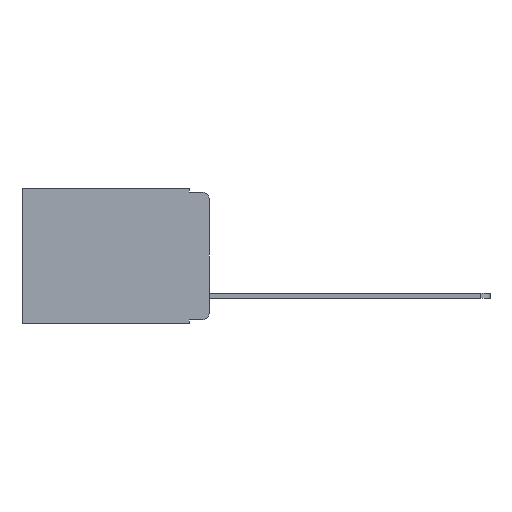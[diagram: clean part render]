
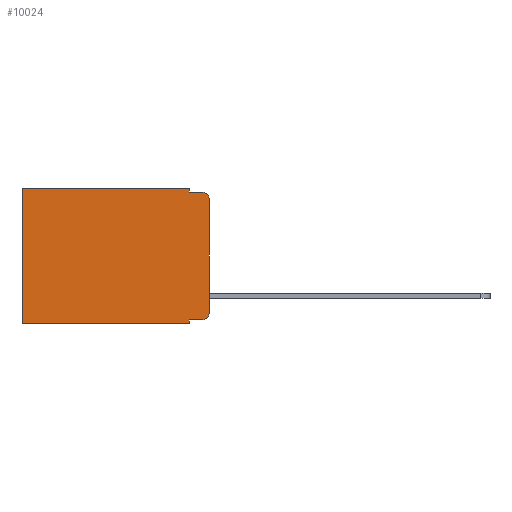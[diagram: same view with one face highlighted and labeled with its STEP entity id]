
A CAD part, left-side view. The second image highlights one B-rep face of the part: STEP entity #10024.
In plain terms, the highlighted planar face has unit normal (-1, 0, 0).
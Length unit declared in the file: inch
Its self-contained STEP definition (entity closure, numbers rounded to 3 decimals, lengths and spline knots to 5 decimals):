
#4 = CARTESIAN_POINT ( 'NONE',  ( 0.298, 0.051, 0. ) ) ;
#123 = VECTOR ( 'NONE', #8739, 39.37008 ) ;
#331 = VECTOR ( 'NONE', #14631, 39.37008 ) ;
#463 = EDGE_CURVE ( 'NONE', #11178, #8515, #7495, .T. ) ;
#680 = VECTOR ( 'NONE', #14620, 39.37008 ) ;
#747 = CARTESIAN_POINT ( 'NONE',  ( 0.298, 0., -0.343 ) ) ;
#1091 = PLANE ( 'NONE',  #6330 ) ;
#1184 = VERTEX_POINT ( 'NONE', #7296 ) ;
#1801 = CARTESIAN_POINT ( 'NONE',  ( 0.298, 0.051, -0.01 ) ) ;
#1900 = DIRECTION ( 'NONE',  ( 0., -1., 0. ) ) ;
#2019 = EDGE_CURVE ( 'NONE', #13394, #2105, #8892, .T. ) ;
#2105 = VERTEX_POINT ( 'NONE', #9127 ) ;
#2339 = VERTEX_POINT ( 'NONE', #5943 ) ;
#2523 = CARTESIAN_POINT ( 'NONE',  ( 0.298, 0.02, -0.333 ) ) ;
#2539 = CARTESIAN_POINT ( 'NONE',  ( 0.298, 0.02, -0.313 ) ) ;
#2757 = CARTESIAN_POINT ( 'NONE',  ( 0.298, 0.473, -0.343 ) ) ;
#3303 = LINE ( 'NONE', #16469, #123 ) ;
#3375 = CARTESIAN_POINT ( 'NONE',  ( 0.298, 0.02, -0.01 ) ) ;
#3895 = DIRECTION ( 'NONE',  ( -1., 0., 0. ) ) ;
#3957 = AXIS2_PLACEMENT_3D ( 'NONE', #2539, #11661, #5196 ) ;
#4052 = CARTESIAN_POINT ( 'NONE',  ( 0.298, 0.02, -0.03 ) ) ;
#4305 = ORIENTED_EDGE ( 'NONE', *, *, #14513, .F. ) ;
#4459 = ORIENTED_EDGE ( 'NONE', *, *, #8218, .F. ) ;
#4557 = EDGE_CURVE ( 'NONE', #2339, #11704, #7590, .T. ) ;
#4608 = EDGE_CURVE ( 'NONE', #1184, #13394, #10288, .T. ) ;
#4707 = ORIENTED_EDGE ( 'NONE', *, *, #5988, .F. ) ;
#4708 = ORIENTED_EDGE ( 'NONE', *, *, #463, .T. ) ;
#4729 = LINE ( 'NONE', #15490, #11447 ) ;
#5196 = DIRECTION ( 'NONE',  ( 0., 0., -1. ) ) ;
#5606 = CARTESIAN_POINT ( 'NONE',  ( 0.298, 0., 0. ) ) ;
#5815 = CARTESIAN_POINT ( 'NONE',  ( 0.298, 0.051, -0.333 ) ) ;
#5943 = CARTESIAN_POINT ( 'NONE',  ( 0.298, 0.051, -0.343 ) ) ;
#5988 = EDGE_CURVE ( 'NONE', #11178, #2105, #3303, .T. ) ;
#6045 = DIRECTION ( 'NONE',  ( 0., 0., -1. ) ) ;
#6305 = VECTOR ( 'NONE', #1900, 39.37008 ) ;
#6330 = AXIS2_PLACEMENT_3D ( 'NONE', #13085, #6538, #15667 ) ;
#6538 = DIRECTION ( 'NONE',  ( 1., 0., 0. ) ) ;
#6628 = DIRECTION ( 'NONE',  ( 0., -1., 0. ) ) ;
#6841 = VECTOR ( 'NONE', #6628, 39.37008 ) ;
#7296 = CARTESIAN_POINT ( 'NONE',  ( 0.298, 0.051, -0.333 ) ) ;
#7348 = EDGE_CURVE ( 'NONE', #1184, #2339, #4729, .T. ) ;
#7431 = VECTOR ( 'NONE', #9685, 39.37008 ) ;
#7495 = CIRCLE ( 'NONE', #14819, 0.02 ) ;
#7590 = LINE ( 'NONE', #747, #331 ) ;
#8218 = EDGE_CURVE ( 'NONE', #12019, #15410, #14430, .T. ) ;
#8515 = VERTEX_POINT ( 'NONE', #3375 ) ;
#8739 = DIRECTION ( 'NONE',  ( 0., 0., -1. ) ) ;
#8892 = CIRCLE ( 'NONE', #3957, 0.02 ) ;
#8944 = ORIENTED_EDGE ( 'NONE', *, *, #10255, .T. ) ;
#9127 = CARTESIAN_POINT ( 'NONE',  ( 0.298, 0., -0.313 ) ) ;
#9151 = ORIENTED_EDGE ( 'NONE', *, *, #15941, .T. ) ;
#9275 = ORIENTED_EDGE ( 'NONE', *, *, #7348, .F. ) ;
#9298 = ORIENTED_EDGE ( 'NONE', *, *, #4557, .F. ) ;
#9323 = CARTESIAN_POINT ( 'NONE',  ( 0.298, 0., -0.03 ) ) ;
#9470 = ORIENTED_EDGE ( 'NONE', *, *, #2019, .T. ) ;
#9685 = DIRECTION ( 'NONE',  ( 0., 1., 0. ) ) ;
#9744 = ORIENTED_EDGE ( 'NONE', *, *, #4608, .T. ) ;
#10024 = ADVANCED_FACE ( 'NONE', ( #10127 ), #1091, .F. ) ;
#10127 = FACE_OUTER_BOUND ( 'NONE', #10191, .T. ) ;
#10191 = EDGE_LOOP ( 'NONE', ( #4707, #4708, #4305, #4459, #9151, #8944, #9298, #9275, #9744, #9470 ) ) ;
#10255 = EDGE_CURVE ( 'NONE', #13640, #11704, #13339, .T. ) ;
#10288 = LINE ( 'NONE', #5815, #6305 ) ;
#10590 = CARTESIAN_POINT ( 'NONE',  ( 0.298, 0.051, -0.01 ) ) ;
#10943 = LINE ( 'NONE', #5606, #7431 ) ;
#11178 = VERTEX_POINT ( 'NONE', #9323 ) ;
#11447 = VECTOR ( 'NONE', #16766, 39.37008 ) ;
#11661 = DIRECTION ( 'NONE',  ( -1., 0., 0. ) ) ;
#11704 = VERTEX_POINT ( 'NONE', #2757 ) ;
#12019 = VERTEX_POINT ( 'NONE', #14089 ) ;
#12338 = CARTESIAN_POINT ( 'NONE',  ( 0.298, 0.473, 0. ) ) ;
#12938 = VECTOR ( 'NONE', #16385, 39.37008 ) ;
#13085 = CARTESIAN_POINT ( 'NONE',  ( 0.298, 0., 0. ) ) ;
#13339 = LINE ( 'NONE', #15104, #12938 ) ;
#13394 = VERTEX_POINT ( 'NONE', #2523 ) ;
#13640 = VERTEX_POINT ( 'NONE', #12338 ) ;
#13825 = LINE ( 'NONE', #10590, #6841 ) ;
#14089 = CARTESIAN_POINT ( 'NONE',  ( 0.298, 0.051, 0. ) ) ;
#14430 = LINE ( 'NONE', #4, #680 ) ;
#14513 = EDGE_CURVE ( 'NONE', #15410, #8515, #13825, .T. ) ;
#14620 = DIRECTION ( 'NONE',  ( 0., 0., -1. ) ) ;
#14631 = DIRECTION ( 'NONE',  ( 0., 1., 0. ) ) ;
#14819 = AXIS2_PLACEMENT_3D ( 'NONE', #4052, #3895, #6045 ) ;
#15104 = CARTESIAN_POINT ( 'NONE',  ( 0.298, 0.473, 0. ) ) ;
#15410 = VERTEX_POINT ( 'NONE', #1801 ) ;
#15490 = CARTESIAN_POINT ( 'NONE',  ( 0.298, 0.051, 0. ) ) ;
#15667 = DIRECTION ( 'NONE',  ( 0., 0., -1. ) ) ;
#15941 = EDGE_CURVE ( 'NONE', #12019, #13640, #10943, .T. ) ;
#16385 = DIRECTION ( 'NONE',  ( 0., 0., -1. ) ) ;
#16469 = CARTESIAN_POINT ( 'NONE',  ( 0.298, 0., 0. ) ) ;
#16766 = DIRECTION ( 'NONE',  ( 0., 0., -1. ) ) ;
